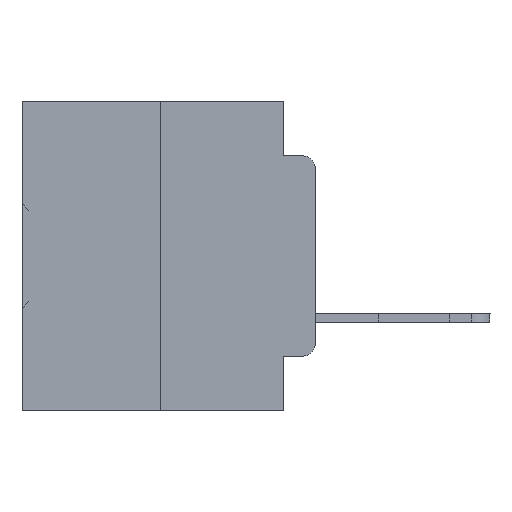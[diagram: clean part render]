
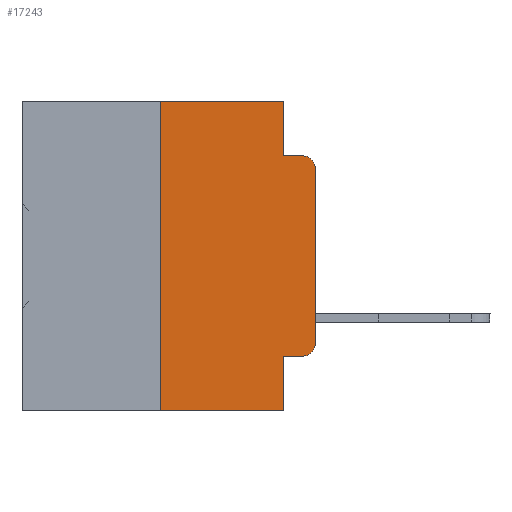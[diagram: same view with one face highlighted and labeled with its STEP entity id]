
A CAD part, left-side view. The second image highlights one B-rep face of the part: STEP entity #17243.
In plain terms, the highlighted planar face has unit normal (-1, 0, 0).
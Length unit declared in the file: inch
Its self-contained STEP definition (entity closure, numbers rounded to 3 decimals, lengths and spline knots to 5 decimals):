
#356 = LINE ( 'NONE', #21444, #16444 ) ;
#472 = EDGE_CURVE ( 'NONE', #6931, #1047, #356, .T. ) ;
#835 = VERTEX_POINT ( 'NONE', #2855 ) ;
#862 = ORIENTED_EDGE ( 'NONE', *, *, #29598, .F. ) ;
#939 = PLANE ( 'NONE',  #36957 ) ;
#1047 = VERTEX_POINT ( 'NONE', #3616 ) ;
#1318 = CARTESIAN_POINT ( 'NONE',  ( 0., 0.473, 0. ) ) ;
#1781 = CARTESIAN_POINT ( 'NONE',  ( 0., 0.051, -0.0885 ) ) ;
#1808 = LINE ( 'NONE', #19209, #6051 ) ;
#2565 = VERTEX_POINT ( 'NONE', #1781 ) ;
#2855 = CARTESIAN_POINT ( 'NONE',  ( 0., 0.051, -0.5 ) ) ;
#3202 = CIRCLE ( 'NONE', #15681, 0.02 ) ;
#3408 = VECTOR ( 'NONE', #12317, 39.37008 ) ;
#3616 = CARTESIAN_POINT ( 'NONE',  ( 0., 0.02, -0.4115 ) ) ;
#3819 = VECTOR ( 'NONE', #25327, 39.37008 ) ;
#4557 = LINE ( 'NONE', #25476, #3408 ) ;
#5242 = LINE ( 'NONE', #6037, #26525 ) ;
#5243 = CIRCLE ( 'NONE', #22762, 0.02 ) ;
#5360 = VECTOR ( 'NONE', #20157, 39.37008 ) ;
#6037 = CARTESIAN_POINT ( 'NONE',  ( 0., 0.473, -0.5 ) ) ;
#6051 = VECTOR ( 'NONE', #31712, 39.37008 ) ;
#6150 = EDGE_CURVE ( 'NONE', #31180, #31213, #19271, .T. ) ;
#6358 = DIRECTION ( 'NONE',  ( -1., 0., 0. ) ) ;
#6931 = VERTEX_POINT ( 'NONE', #10193 ) ;
#8735 = CARTESIAN_POINT ( 'NONE',  ( 0., 0.02, -0.0885 ) ) ;
#9012 = EDGE_CURVE ( 'NONE', #31180, #835, #5242, .T. ) ;
#9057 = ORIENTED_EDGE ( 'NONE', *, *, #16320, .T. ) ;
#9266 = ORIENTED_EDGE ( 'NONE', *, *, #26603, .F. ) ;
#9309 = DIRECTION ( 'NONE',  ( 0., 0., -1. ) ) ;
#9914 = CARTESIAN_POINT ( 'NONE',  ( 0., 0.25, 0. ) ) ;
#10193 = CARTESIAN_POINT ( 'NONE',  ( 0., 0.051, -0.4115 ) ) ;
#10445 = EDGE_CURVE ( 'NONE', #14671, #36870, #35615, .T. ) ;
#11355 = VECTOR ( 'NONE', #9309, 39.37008 ) ;
#11544 = EDGE_CURVE ( 'NONE', #15425, #2565, #1808, .T. ) ;
#12046 = CARTESIAN_POINT ( 'NONE',  ( 0., 0.051, 0. ) ) ;
#12203 = ORIENTED_EDGE ( 'NONE', *, *, #21438, .F. ) ;
#12317 = DIRECTION ( 'NONE',  ( 0., -1., 0. ) ) ;
#13229 = FACE_OUTER_BOUND ( 'NONE', #20231, .T. ) ;
#14671 = VERTEX_POINT ( 'NONE', #33015 ) ;
#15425 = VERTEX_POINT ( 'NONE', #20554 ) ;
#15681 = AXIS2_PLACEMENT_3D ( 'NONE', #30411, #6358, #24545 ) ;
#15710 = LINE ( 'NONE', #24718, #19279 ) ;
#15757 = CARTESIAN_POINT ( 'NONE',  ( 0., 0.25, 0. ) ) ;
#15790 = ORIENTED_EDGE ( 'NONE', *, *, #37917, .T. ) ;
#16320 = EDGE_CURVE ( 'NONE', #1047, #14671, #3202, .T. ) ;
#16444 = VECTOR ( 'NONE', #35758, 39.37008 ) ;
#17243 = ADVANCED_FACE ( 'NONE', ( #13229 ), #939, .F. ) ;
#19209 = CARTESIAN_POINT ( 'NONE',  ( 0., 0.051, 0. ) ) ;
#19271 = LINE ( 'NONE', #15757, #3819 ) ;
#19279 = VECTOR ( 'NONE', #36463, 39.37008 ) ;
#19847 = ORIENTED_EDGE ( 'NONE', *, *, #472, .T. ) ;
#20157 = DIRECTION ( 'NONE',  ( 0., 0., 1. ) ) ;
#20231 = EDGE_LOOP ( 'NONE', ( #27231, #15790, #12203, #35822, #9266, #28551, #37053, #862, #19847, #9057 ) ) ;
#20554 = CARTESIAN_POINT ( 'NONE',  ( 0., 0.051, 0. ) ) ;
#21438 = EDGE_CURVE ( 'NONE', #2565, #29335, #4557, .T. ) ;
#21444 = CARTESIAN_POINT ( 'NONE',  ( 0., 0.051, -0.4115 ) ) ;
#22762 = AXIS2_PLACEMENT_3D ( 'NONE', #28658, #31783, #22999 ) ;
#22999 = DIRECTION ( 'NONE',  ( 0., 0., -1. ) ) ;
#23294 = CARTESIAN_POINT ( 'NONE',  ( 0., 0., 0. ) ) ;
#24202 = CARTESIAN_POINT ( 'NONE',  ( 0., 0.25, -0.5 ) ) ;
#24545 = DIRECTION ( 'NONE',  ( 0., 0., -1. ) ) ;
#24600 = DIRECTION ( 'NONE',  ( 1., 0., 0. ) ) ;
#24718 = CARTESIAN_POINT ( 'NONE',  ( 0., 0.473, 0. ) ) ;
#25327 = DIRECTION ( 'NONE',  ( 0., 0., 1. ) ) ;
#25476 = CARTESIAN_POINT ( 'NONE',  ( 0., 0.051, -0.0885 ) ) ;
#26525 = VECTOR ( 'NONE', #29693, 39.37008 ) ;
#26603 = EDGE_CURVE ( 'NONE', #31213, #15425, #15710, .T. ) ;
#27231 = ORIENTED_EDGE ( 'NONE', *, *, #10445, .T. ) ;
#28551 = ORIENTED_EDGE ( 'NONE', *, *, #6150, .F. ) ;
#28658 = CARTESIAN_POINT ( 'NONE',  ( 0., 0.02, -0.1085 ) ) ;
#29335 = VERTEX_POINT ( 'NONE', #8735 ) ;
#29598 = EDGE_CURVE ( 'NONE', #6931, #835, #36480, .T. ) ;
#29693 = DIRECTION ( 'NONE',  ( 0., -1., 0. ) ) ;
#30167 = CARTESIAN_POINT ( 'NONE',  ( 0., 0., -0.1085 ) ) ;
#30411 = CARTESIAN_POINT ( 'NONE',  ( 0., 0.02, -0.3915 ) ) ;
#31180 = VERTEX_POINT ( 'NONE', #24202 ) ;
#31213 = VERTEX_POINT ( 'NONE', #9914 ) ;
#31712 = DIRECTION ( 'NONE',  ( 0., 0., -1. ) ) ;
#31783 = DIRECTION ( 'NONE',  ( -1., 0., 0. ) ) ;
#33015 = CARTESIAN_POINT ( 'NONE',  ( 0., 0., -0.3915 ) ) ;
#33976 = DIRECTION ( 'NONE',  ( 0., 0., -1. ) ) ;
#35615 = LINE ( 'NONE', #23294, #5360 ) ;
#35758 = DIRECTION ( 'NONE',  ( 0., -1., 0. ) ) ;
#35822 = ORIENTED_EDGE ( 'NONE', *, *, #11544, .F. ) ;
#36463 = DIRECTION ( 'NONE',  ( 0., -1., 0. ) ) ;
#36480 = LINE ( 'NONE', #12046, #11355 ) ;
#36870 = VERTEX_POINT ( 'NONE', #30167 ) ;
#36957 = AXIS2_PLACEMENT_3D ( 'NONE', #1318, #24600, #33976 ) ;
#37053 = ORIENTED_EDGE ( 'NONE', *, *, #9012, .T. ) ;
#37917 = EDGE_CURVE ( 'NONE', #36870, #29335, #5243, .T. ) ;
